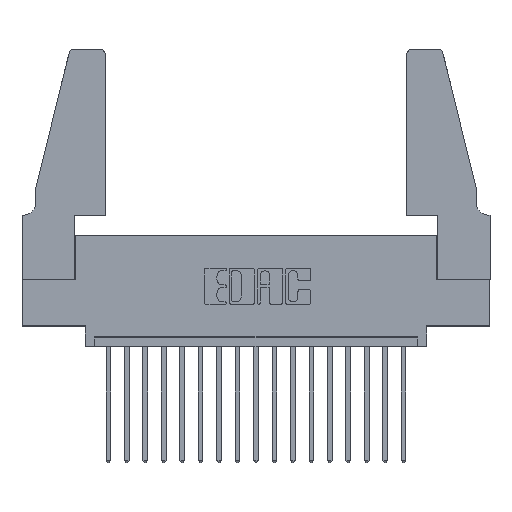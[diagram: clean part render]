
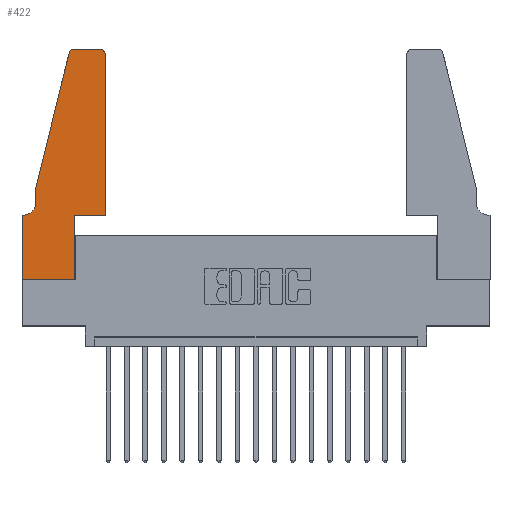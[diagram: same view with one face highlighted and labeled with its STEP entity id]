
A CAD part, top view. The second image highlights one B-rep face of the part: STEP entity #422.
In plain terms, the highlighted planar face has unit normal (0, 0, 1).
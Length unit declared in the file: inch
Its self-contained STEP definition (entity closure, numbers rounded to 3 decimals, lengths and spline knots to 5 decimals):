
#169 = EDGE_CURVE ( 'NONE', #17099, #7777, #13324, .T. ) ;
#422 = ADVANCED_FACE ( 'NONE', ( #18433 ), #6787, .T. ) ;
#542 = CARTESIAN_POINT ( 'NONE',  ( 0.4205, 1.25, 0.37 ) ) ;
#597 = EDGE_CURVE ( 'NONE', #4977, #7045, #4171, .T. ) ;
#690 = CARTESIAN_POINT ( 'NONE',  ( 0., 0., 0.37 ) ) ;
#698 = DIRECTION ( 'NONE',  ( 0., -1., 0. ) ) ;
#1044 = EDGE_CURVE ( 'NONE', #6319, #10517, #9331, .T. ) ;
#1069 = CARTESIAN_POINT ( 'NONE',  ( 0., 0.35, 0.37 ) ) ;
#1500 = LINE ( 'NONE', #4850, #15558 ) ;
#1637 = CARTESIAN_POINT ( 'NONE',  ( 0.2865, 0.35, 0.37 ) ) ;
#1905 = EDGE_LOOP ( 'NONE', ( #5921, #13180, #18372, #12153, #6271, #17429, #17146, #15382, #14683, #4150, #17662, #4424 ) ) ;
#2448 = DIRECTION ( 'NONE',  ( 1., 0., 0. ) ) ;
#2910 = DIRECTION ( 'NONE',  ( 0., -1., 0. ) ) ;
#3426 = CARTESIAN_POINT ( 'NONE',  ( 0.2865, 0., 0.37 ) ) ;
#3560 = LINE ( 'NONE', #6328, #10061 ) ;
#3695 = DIRECTION ( 'NONE',  ( 0., 0., 1. ) ) ;
#3971 = LINE ( 'NONE', #1637, #4894 ) ;
#4150 = ORIENTED_EDGE ( 'NONE', *, *, #17475, .T. ) ;
#4171 = LINE ( 'NONE', #13771, #5990 ) ;
#4424 = ORIENTED_EDGE ( 'NONE', *, *, #7449, .T. ) ;
#4850 = CARTESIAN_POINT ( 'NONE',  ( 0., 0., 0.37 ) ) ;
#4894 = VECTOR ( 'NONE', #10295, 39.37008 ) ;
#4977 = VERTEX_POINT ( 'NONE', #14599 ) ;
#5069 = CIRCLE ( 'NONE', #15839, 0.07 ) ;
#5084 = LINE ( 'NONE', #5738, #9774 ) ;
#5107 = CIRCLE ( 'NONE', #5335, 0.03 ) ;
#5238 = EDGE_CURVE ( 'NONE', #6934, #14248, #3971, .T. ) ;
#5240 = DIRECTION ( 'NONE',  ( -0.239, -0.971, 0. ) ) ;
#5335 = AXIS2_PLACEMENT_3D ( 'NONE', #8122, #3695, #2448 ) ;
#5384 = CARTESIAN_POINT ( 'NONE',  ( 0.0055, 0.42, 0.37 ) ) ;
#5419 = CARTESIAN_POINT ( 'NONE',  ( 0.4505, 1.22, 0.37 ) ) ;
#5738 = CARTESIAN_POINT ( 'NONE',  ( 0.4505, 0.35, 0.37 ) ) ;
#5819 = CARTESIAN_POINT ( 'NONE',  ( 0.0755, 0.5, 0.37 ) ) ;
#5921 = ORIENTED_EDGE ( 'NONE', *, *, #15151, .T. ) ;
#5990 = VECTOR ( 'NONE', #5240, 39.37008 ) ;
#6131 = DIRECTION ( 'NONE',  ( -1., 0., 0. ) ) ;
#6165 = CARTESIAN_POINT ( 'NONE',  ( 0.0055, 0.35, 0.37 ) ) ;
#6195 = DIRECTION ( 'NONE',  ( 1., 0., 0. ) ) ;
#6228 = VECTOR ( 'NONE', #13213, 39.37008 ) ;
#6271 = ORIENTED_EDGE ( 'NONE', *, *, #9003, .T. ) ;
#6319 = VERTEX_POINT ( 'NONE', #6165 ) ;
#6328 = CARTESIAN_POINT ( 'NONE',  ( 0.2605, 1.25, 0.37 ) ) ;
#6785 = CARTESIAN_POINT ( 'NONE',  ( 0.284, 1.25, 0.37 ) ) ;
#6787 = PLANE ( 'NONE',  #14229 ) ;
#6864 = VERTEX_POINT ( 'NONE', #17593 ) ;
#6934 = VERTEX_POINT ( 'NONE', #3426 ) ;
#7045 = VERTEX_POINT ( 'NONE', #7793 ) ;
#7449 = EDGE_CURVE ( 'NONE', #7777, #17975, #10276, .T. ) ;
#7633 = CARTESIAN_POINT ( 'NONE',  ( 0., 0.35, 0.37 ) ) ;
#7777 = VERTEX_POINT ( 'NONE', #5419 ) ;
#7793 = CARTESIAN_POINT ( 'NONE',  ( 0.0755, 0.5, 0.37 ) ) ;
#7812 = CARTESIAN_POINT ( 'NONE',  ( 0., 0., 0.37 ) ) ;
#8122 = CARTESIAN_POINT ( 'NONE',  ( 0.284, 1.22, 0.37 ) ) ;
#8143 = EDGE_CURVE ( 'NONE', #10517, #13770, #12276, .T. ) ;
#8165 = EDGE_CURVE ( 'NONE', #13770, #6934, #1500, .T. ) ;
#8291 = VERTEX_POINT ( 'NONE', #6785 ) ;
#9003 = EDGE_CURVE ( 'NONE', #6864, #6319, #5069, .T. ) ;
#9331 = LINE ( 'NONE', #9802, #15302 ) ;
#9697 = DIRECTION ( 'NONE',  ( -1., 0., 0. ) ) ;
#9774 = VECTOR ( 'NONE', #10055, 39.37008 ) ;
#9802 = CARTESIAN_POINT ( 'NONE',  ( 0.0755, 0.35, 0.37 ) ) ;
#10055 = DIRECTION ( 'NONE',  ( 1., 0., 0. ) ) ;
#10061 = VECTOR ( 'NONE', #6131, 39.37008 ) ;
#10276 = CIRCLE ( 'NONE', #11573, 0.03 ) ;
#10295 = DIRECTION ( 'NONE',  ( 0., 1., 0. ) ) ;
#10347 = CARTESIAN_POINT ( 'NONE',  ( 0.4505, 0.35, 0.37 ) ) ;
#10477 = DIRECTION ( 'NONE',  ( -1., 0., 0. ) ) ;
#10517 = VERTEX_POINT ( 'NONE', #7633 ) ;
#10821 = CARTESIAN_POINT ( 'NONE',  ( 0.4505, 0.35, 0.37 ) ) ;
#11026 = DIRECTION ( 'NONE',  ( 0., 0., 1. ) ) ;
#11573 = AXIS2_PLACEMENT_3D ( 'NONE', #13529, #13290, #6195 ) ;
#12153 = ORIENTED_EDGE ( 'NONE', *, *, #15628, .T. ) ;
#12276 = LINE ( 'NONE', #7812, #14895 ) ;
#13180 = ORIENTED_EDGE ( 'NONE', *, *, #16593, .T. ) ;
#13213 = DIRECTION ( 'NONE',  ( 0., 1., 0. ) ) ;
#13290 = DIRECTION ( 'NONE',  ( 0., 0., 1. ) ) ;
#13324 = LINE ( 'NONE', #10347, #6228 ) ;
#13529 = CARTESIAN_POINT ( 'NONE',  ( 0.4205, 1.22, 0.37 ) ) ;
#13770 = VERTEX_POINT ( 'NONE', #690 ) ;
#13771 = CARTESIAN_POINT ( 'NONE',  ( 0.0755, 0.5, 0.37 ) ) ;
#14229 = AXIS2_PLACEMENT_3D ( 'NONE', #1069, #11026, #15348 ) ;
#14248 = VERTEX_POINT ( 'NONE', #17261 ) ;
#14599 = CARTESIAN_POINT ( 'NONE',  ( 0.25487, 1.22718, 0.37 ) ) ;
#14683 = ORIENTED_EDGE ( 'NONE', *, *, #5238, .T. ) ;
#14895 = VECTOR ( 'NONE', #698, 39.37008 ) ;
#15151 = EDGE_CURVE ( 'NONE', #17975, #8291, #3560, .T. ) ;
#15302 = VECTOR ( 'NONE', #10477, 39.37008 ) ;
#15348 = DIRECTION ( 'NONE',  ( 1., 0., 0. ) ) ;
#15382 = ORIENTED_EDGE ( 'NONE', *, *, #8165, .T. ) ;
#15558 = VECTOR ( 'NONE', #16357, 39.37008 ) ;
#15628 = EDGE_CURVE ( 'NONE', #7045, #6864, #18025, .T. ) ;
#15839 = AXIS2_PLACEMENT_3D ( 'NONE', #5384, #18192, #9697 ) ;
#16357 = DIRECTION ( 'NONE',  ( 1., 0., 0. ) ) ;
#16465 = VECTOR ( 'NONE', #2910, 39.37008 ) ;
#16593 = EDGE_CURVE ( 'NONE', #8291, #4977, #5107, .T. ) ;
#17099 = VERTEX_POINT ( 'NONE', #10821 ) ;
#17146 = ORIENTED_EDGE ( 'NONE', *, *, #8143, .T. ) ;
#17261 = CARTESIAN_POINT ( 'NONE',  ( 0.2865, 0.35, 0.37 ) ) ;
#17429 = ORIENTED_EDGE ( 'NONE', *, *, #1044, .T. ) ;
#17475 = EDGE_CURVE ( 'NONE', #14248, #17099, #5084, .T. ) ;
#17593 = CARTESIAN_POINT ( 'NONE',  ( 0.0755, 0.42, 0.37 ) ) ;
#17662 = ORIENTED_EDGE ( 'NONE', *, *, #169, .T. ) ;
#17975 = VERTEX_POINT ( 'NONE', #542 ) ;
#18025 = LINE ( 'NONE', #5819, #16465 ) ;
#18192 = DIRECTION ( 'NONE',  ( 0., 0., -1. ) ) ;
#18372 = ORIENTED_EDGE ( 'NONE', *, *, #597, .T. ) ;
#18433 = FACE_OUTER_BOUND ( 'NONE', #1905, .T. ) ;
